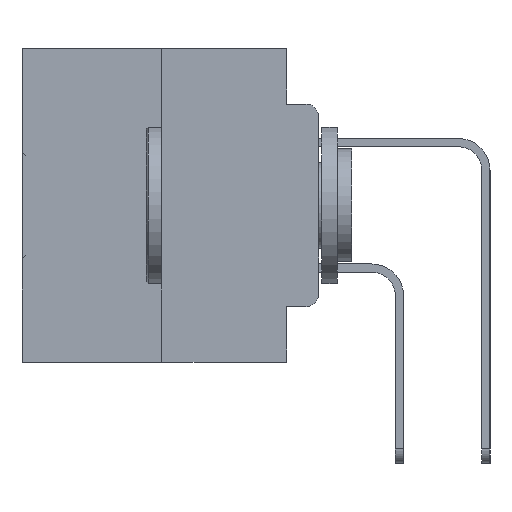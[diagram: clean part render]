
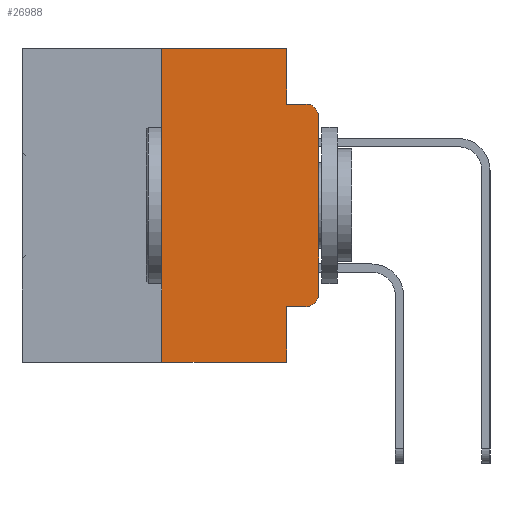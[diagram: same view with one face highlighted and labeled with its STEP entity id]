
A CAD part, left-side view. The second image highlights one B-rep face of the part: STEP entity #26988.
In plain terms, the highlighted planar face has unit normal (-1, 0, 0).
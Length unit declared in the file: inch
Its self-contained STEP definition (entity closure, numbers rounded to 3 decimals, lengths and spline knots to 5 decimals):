
#1002 = CARTESIAN_POINT ( 'NONE',  ( 0., 0.25, -0.5 ) ) ;
#1050 = CARTESIAN_POINT ( 'NONE',  ( 0., 0., -0.1085 ) ) ;
#1173 = EDGE_LOOP ( 'NONE', ( #23356, #32546, #19741, #24579, #26200, #27015, #20192, #33206, #15209, #13211 ) ) ;
#1180 = VERTEX_POINT ( 'NONE', #28274 ) ;
#1293 = CARTESIAN_POINT ( 'NONE',  ( 0., 0.051, 0. ) ) ;
#1524 = AXIS2_PLACEMENT_3D ( 'NONE', #25280, #9861, #27881 ) ;
#1621 = CARTESIAN_POINT ( 'NONE',  ( 0., 0., 0. ) ) ;
#1815 = DIRECTION ( 'NONE',  ( 0., -1., 0. ) ) ;
#2403 = VECTOR ( 'NONE', #29267, 39.37008 ) ;
#3363 = EDGE_CURVE ( 'NONE', #4955, #1180, #13417, .T. ) ;
#3613 = VECTOR ( 'NONE', #29902, 39.37008 ) ;
#3907 = DIRECTION ( 'NONE',  ( 0., 0., -1. ) ) ;
#4955 = VERTEX_POINT ( 'NONE', #1050 ) ;
#5109 = EDGE_CURVE ( 'NONE', #24398, #4955, #18144, .T. ) ;
#5338 = CARTESIAN_POINT ( 'NONE',  ( 0., 0.02, -0.3915 ) ) ;
#5608 = DIRECTION ( 'NONE',  ( 0., 0., -1. ) ) ;
#5753 = LINE ( 'NONE', #29490, #19448 ) ;
#6239 = AXIS2_PLACEMENT_3D ( 'NONE', #31223, #21021, #5608 ) ;
#6335 = AXIS2_PLACEMENT_3D ( 'NONE', #5338, #23345, #7932 ) ;
#6384 = VERTEX_POINT ( 'NONE', #17861 ) ;
#6531 = LINE ( 'NONE', #1293, #19428 ) ;
#7932 = DIRECTION ( 'NONE',  ( 0., 0., -1. ) ) ;
#9861 = DIRECTION ( 'NONE',  ( -1., 0., 0. ) ) ;
#10102 = LINE ( 'NONE', #13883, #2403 ) ;
#11185 = EDGE_CURVE ( 'NONE', #19197, #6384, #26284, .T. ) ;
#12064 = CARTESIAN_POINT ( 'NONE',  ( 0., 0.051, -0.0885 ) ) ;
#13187 = DIRECTION ( 'NONE',  ( 0., -1., 0. ) ) ;
#13211 = ORIENTED_EDGE ( 'NONE', *, *, #21279, .T. ) ;
#13417 = CIRCLE ( 'NONE', #1524, 0.02 ) ;
#13883 = CARTESIAN_POINT ( 'NONE',  ( 0., 0.25, 0. ) ) ;
#14080 = DIRECTION ( 'NONE',  ( 0., 0., -1. ) ) ;
#14099 = LINE ( 'NONE', #12064, #26967 ) ;
#14519 = FACE_OUTER_BOUND ( 'NONE', #1173, .T. ) ;
#14663 = DIRECTION ( 'NONE',  ( 0., -1., 0. ) ) ;
#15060 = DIRECTION ( 'NONE',  ( 0., -1., 0. ) ) ;
#15209 = ORIENTED_EDGE ( 'NONE', *, *, #23006, .T. ) ;
#16139 = CIRCLE ( 'NONE', #6335, 0.02 ) ;
#16871 = VERTEX_POINT ( 'NONE', #21204 ) ;
#16924 = VECTOR ( 'NONE', #13187, 39.37008 ) ;
#16952 = VERTEX_POINT ( 'NONE', #1002 ) ;
#17136 = CARTESIAN_POINT ( 'NONE',  ( 0., 0.051, -0.5 ) ) ;
#17201 = VERTEX_POINT ( 'NONE', #25230 ) ;
#17861 = CARTESIAN_POINT ( 'NONE',  ( 0., 0.051, 0. ) ) ;
#17940 = LINE ( 'NONE', #32613, #30785 ) ;
#18144 = LINE ( 'NONE', #1621, #3613 ) ;
#19197 = VERTEX_POINT ( 'NONE', #26917 ) ;
#19428 = VECTOR ( 'NONE', #3907, 39.37008 ) ;
#19448 = VECTOR ( 'NONE', #14080, 39.37008 ) ;
#19741 = ORIENTED_EDGE ( 'NONE', *, *, #33277, .F. ) ;
#20192 = ORIENTED_EDGE ( 'NONE', *, *, #26916, .T. ) ;
#20906 = PLANE ( 'NONE',  #6239 ) ;
#21021 = DIRECTION ( 'NONE',  ( 1., 0., 0. ) ) ;
#21204 = CARTESIAN_POINT ( 'NONE',  ( 0., 0.051, -0.4115 ) ) ;
#21279 = EDGE_CURVE ( 'NONE', #28951, #24398, #16139, .T. ) ;
#21473 = CARTESIAN_POINT ( 'NONE',  ( 0., 0.02, -0.4115 ) ) ;
#22667 = CARTESIAN_POINT ( 'NONE',  ( 0., 0.473, 0. ) ) ;
#22950 = LINE ( 'NONE', #28577, #16924 ) ;
#23006 = EDGE_CURVE ( 'NONE', #16871, #28951, #17940, .T. ) ;
#23191 = CARTESIAN_POINT ( 'NONE',  ( 0., 0., -0.3915 ) ) ;
#23345 = DIRECTION ( 'NONE',  ( -1., 0., 0. ) ) ;
#23356 = ORIENTED_EDGE ( 'NONE', *, *, #5109, .T. ) ;
#24398 = VERTEX_POINT ( 'NONE', #23191 ) ;
#24579 = ORIENTED_EDGE ( 'NONE', *, *, #31593, .F. ) ;
#24736 = EDGE_CURVE ( 'NONE', #16871, #26025, #6531, .T. ) ;
#25230 = CARTESIAN_POINT ( 'NONE',  ( 0., 0.051, -0.0885 ) ) ;
#25280 = CARTESIAN_POINT ( 'NONE',  ( 0., 0.02, -0.1085 ) ) ;
#26025 = VERTEX_POINT ( 'NONE', #17136 ) ;
#26200 = ORIENTED_EDGE ( 'NONE', *, *, #11185, .F. ) ;
#26284 = LINE ( 'NONE', #22667, #32238 ) ;
#26463 = EDGE_CURVE ( 'NONE', #16952, #19197, #10102, .T. ) ;
#26916 = EDGE_CURVE ( 'NONE', #16952, #26025, #22950, .T. ) ;
#26917 = CARTESIAN_POINT ( 'NONE',  ( 0., 0.25, 0. ) ) ;
#26967 = VECTOR ( 'NONE', #14663, 39.37008 ) ;
#26988 = ADVANCED_FACE ( 'NONE', ( #14519 ), #20906, .F. ) ;
#27015 = ORIENTED_EDGE ( 'NONE', *, *, #26463, .F. ) ;
#27881 = DIRECTION ( 'NONE',  ( 0., 0., -1. ) ) ;
#28274 = CARTESIAN_POINT ( 'NONE',  ( 0., 0.02, -0.0885 ) ) ;
#28577 = CARTESIAN_POINT ( 'NONE',  ( 0., 0.473, -0.5 ) ) ;
#28951 = VERTEX_POINT ( 'NONE', #21473 ) ;
#29267 = DIRECTION ( 'NONE',  ( 0., 0., 1. ) ) ;
#29490 = CARTESIAN_POINT ( 'NONE',  ( 0., 0.051, 0. ) ) ;
#29902 = DIRECTION ( 'NONE',  ( 0., 0., 1. ) ) ;
#30785 = VECTOR ( 'NONE', #1815, 39.37008 ) ;
#31223 = CARTESIAN_POINT ( 'NONE',  ( 0., 0.473, 0. ) ) ;
#31593 = EDGE_CURVE ( 'NONE', #6384, #17201, #5753, .T. ) ;
#32238 = VECTOR ( 'NONE', #15060, 39.37008 ) ;
#32546 = ORIENTED_EDGE ( 'NONE', *, *, #3363, .T. ) ;
#32613 = CARTESIAN_POINT ( 'NONE',  ( 0., 0.051, -0.4115 ) ) ;
#33206 = ORIENTED_EDGE ( 'NONE', *, *, #24736, .F. ) ;
#33277 = EDGE_CURVE ( 'NONE', #17201, #1180, #14099, .T. ) ;
